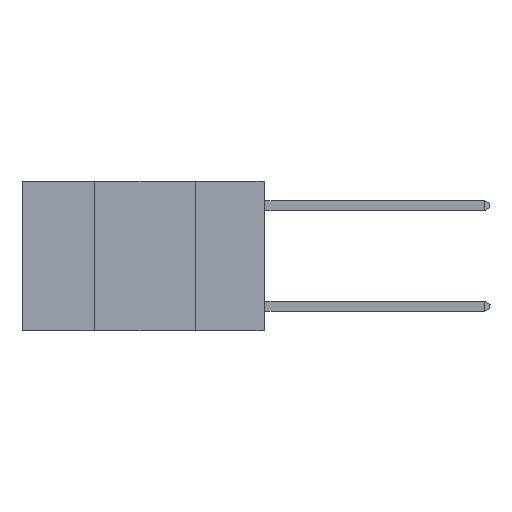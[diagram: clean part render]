
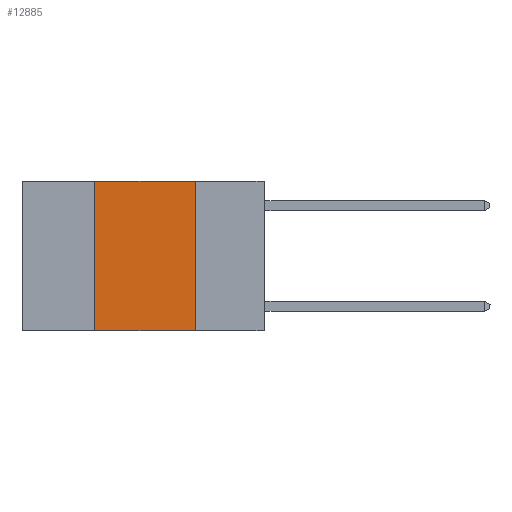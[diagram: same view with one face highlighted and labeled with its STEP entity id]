
A CAD part, left-side view. The second image highlights one B-rep face of the part: STEP entity #12885.
In plain terms, the highlighted planar face has unit normal (-1, 0, 0).
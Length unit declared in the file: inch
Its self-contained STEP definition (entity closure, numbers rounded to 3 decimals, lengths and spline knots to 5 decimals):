
#83 = CARTESIAN_POINT ( 'NONE',  ( 0., 0.42, 0. ) ) ;
#827 = EDGE_CURVE ( 'NONE', #1348, #6807, #5434, .T. ) ;
#1047 = ORIENTED_EDGE ( 'NONE', *, *, #11593, .F. ) ;
#1143 = FACE_OUTER_BOUND ( 'NONE', #8978, .T. ) ;
#1348 = VERTEX_POINT ( 'NONE', #83 ) ;
#1555 = DIRECTION ( 'NONE',  ( 0., 0., 1. ) ) ;
#1556 = CARTESIAN_POINT ( 'NONE',  ( 0., 0.6, 0. ) ) ;
#1955 = PLANE ( 'NONE',  #9759 ) ;
#3035 = CARTESIAN_POINT ( 'NONE',  ( 0., 0.17, 0. ) ) ;
#3162 = LINE ( 'NONE', #14763, #6208 ) ;
#4127 = DIRECTION ( 'NONE',  ( 0., 0., -1. ) ) ;
#4467 = ORIENTED_EDGE ( 'NONE', *, *, #11136, .T. ) ;
#5173 = CARTESIAN_POINT ( 'NONE',  ( 0., 0.42, -0.37 ) ) ;
#5278 = CARTESIAN_POINT ( 'NONE',  ( 0., 0.17, 0. ) ) ;
#5416 = DIRECTION ( 'NONE',  ( 1., 0., 0. ) ) ;
#5434 = LINE ( 'NONE', #1556, #8106 ) ;
#6208 = VECTOR ( 'NONE', #12454, 39.37008 ) ;
#6807 = VERTEX_POINT ( 'NONE', #3035 ) ;
#7263 = DIRECTION ( 'NONE',  ( 0., -1., 0. ) ) ;
#8106 = VECTOR ( 'NONE', #7263, 39.37008 ) ;
#8511 = LINE ( 'NONE', #5278, #11878 ) ;
#8791 = CARTESIAN_POINT ( 'NONE',  ( 0., 0.6, 0. ) ) ;
#8978 = EDGE_LOOP ( 'NONE', ( #1047, #10135, #13177, #4467 ) ) ;
#9119 = VERTEX_POINT ( 'NONE', #10561 ) ;
#9142 = EDGE_CURVE ( 'NONE', #13393, #1348, #11762, .T. ) ;
#9759 = AXIS2_PLACEMENT_3D ( 'NONE', #8791, #5416, #13355 ) ;
#10135 = ORIENTED_EDGE ( 'NONE', *, *, #827, .F. ) ;
#10561 = CARTESIAN_POINT ( 'NONE',  ( 0., 0.17, -0.37 ) ) ;
#10654 = CARTESIAN_POINT ( 'NONE',  ( 0., 0.42, 0. ) ) ;
#11136 = EDGE_CURVE ( 'NONE', #13393, #9119, #3162, .T. ) ;
#11593 = EDGE_CURVE ( 'NONE', #6807, #9119, #8511, .T. ) ;
#11762 = LINE ( 'NONE', #10654, #14437 ) ;
#11878 = VECTOR ( 'NONE', #4127, 39.37008 ) ;
#12454 = DIRECTION ( 'NONE',  ( 0., -1., 0. ) ) ;
#12885 = ADVANCED_FACE ( 'NONE', ( #1143 ), #1955, .F. ) ;
#13177 = ORIENTED_EDGE ( 'NONE', *, *, #9142, .F. ) ;
#13355 = DIRECTION ( 'NONE',  ( 0., 0., -1. ) ) ;
#13393 = VERTEX_POINT ( 'NONE', #5173 ) ;
#14437 = VECTOR ( 'NONE', #1555, 39.37008 ) ;
#14763 = CARTESIAN_POINT ( 'NONE',  ( 0., 0.6, -0.37 ) ) ;
